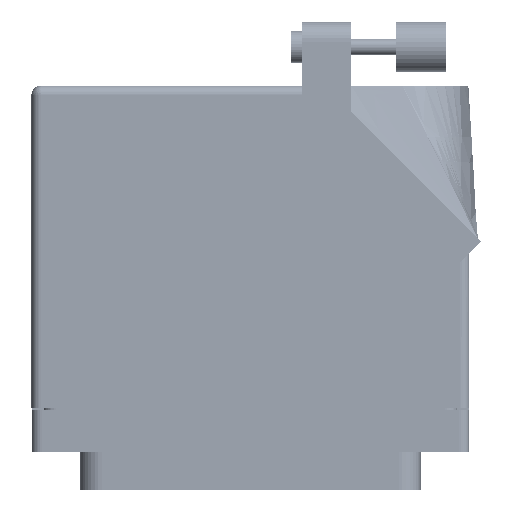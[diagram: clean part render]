
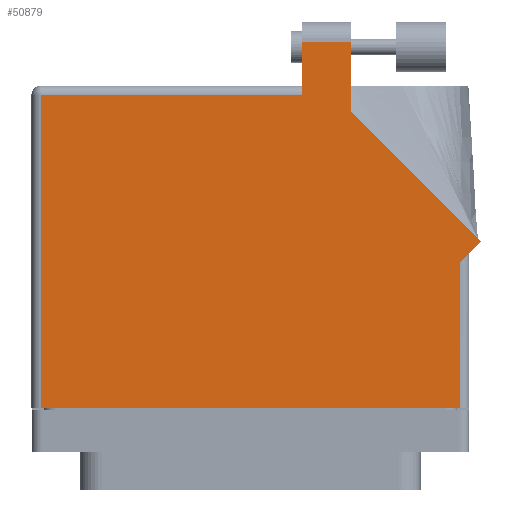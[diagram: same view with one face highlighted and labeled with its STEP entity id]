
A CAD part, front view. The second image highlights one B-rep face of the part: STEP entity #50879.
In plain terms, the highlighted face is planar.
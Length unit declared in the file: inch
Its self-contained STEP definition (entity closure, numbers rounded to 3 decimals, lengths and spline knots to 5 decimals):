
#1289 = VECTOR ( 'NONE', #21052, 39.37008 ) ;
#1736 = DIRECTION ( 'NONE',  ( 0., 1., 0. ) ) ;
#1799 = CARTESIAN_POINT ( 'NONE',  ( -1.3155, -0.1, 0.765 ) ) ;
#4821 = EDGE_CURVE ( 'NONE', #65087, #63755, #14002, .T. ) ;
#5730 = ORIENTED_EDGE ( 'NONE', *, *, #4821, .T. ) ;
#5805 = DIRECTION ( 'NONE',  ( -1., 0., 0. ) ) ;
#8644 = CARTESIAN_POINT ( 'NONE',  ( 0.6345, 1.76442, 0.765 ) ) ;
#9148 = VECTOR ( 'NONE', #45414, 39.37008 ) ;
#10805 = VERTEX_POINT ( 'NONE', #79497 ) ;
#12740 = LINE ( 'NONE', #88213, #39972 ) ;
#12773 = EDGE_CURVE ( 'NONE', #34754, #37723, #15149, .T. ) ;
#13889 = LINE ( 'NONE', #42337, #24087 ) ;
#14002 = LINE ( 'NONE', #1799, #28987 ) ;
#15149 = LINE ( 'NONE', #49030, #1289 ) ;
#16421 = EDGE_CURVE ( 'NONE', #44333, #29971, #66097, .T. ) ;
#19986 = CARTESIAN_POINT ( 'NONE',  ( -1.3155, -0.1, 0.765 ) ) ;
#21052 = DIRECTION ( 'NONE',  ( 0.707, 0.707, 0. ) ) ;
#21336 = CARTESIAN_POINT ( 'NONE',  ( -1.3155, 1.868, 0.765 ) ) ;
#22315 = ORIENTED_EDGE ( 'NONE', *, *, #12773, .T. ) ;
#22986 = LINE ( 'NONE', #49618, #57344 ) ;
#23316 = VECTOR ( 'NONE', #5805, 39.37008 ) ;
#23936 = CARTESIAN_POINT ( 'NONE',  ( 0.6345, 1.76442, 0.765 ) ) ;
#24087 = VECTOR ( 'NONE', #69951, 39.37008 ) ;
#27228 = DIRECTION ( 'NONE',  ( -1., 0., 0. ) ) ;
#28310 = VERTEX_POINT ( 'NONE', #46020 ) ;
#28943 = ORIENTED_EDGE ( 'NONE', *, *, #55375, .T. ) ;
#28987 = VECTOR ( 'NONE', #63258, 39.37008 ) ;
#29317 = LINE ( 'NONE', #36082, #59808 ) ;
#29971 = VERTEX_POINT ( 'NONE', #63590 ) ;
#33529 = CARTESIAN_POINT ( 'NONE',  ( -1.3775, 1.93, 0.765 ) ) ;
#34754 = VERTEX_POINT ( 'NONE', #73357 ) ;
#36082 = CARTESIAN_POINT ( 'NONE',  ( 1.3155, 0.88, 0.765 ) ) ;
#37723 = VERTEX_POINT ( 'NONE', #46540 ) ;
#39326 = VECTOR ( 'NONE', #43794, 39.37008 ) ;
#39972 = VECTOR ( 'NONE', #27228, 39.37008 ) ;
#42337 = CARTESIAN_POINT ( 'NONE',  ( 0.3275, 1.93, 0.765 ) ) ;
#42959 = EDGE_CURVE ( 'NONE', #29971, #10805, #13889, .T. ) ;
#43794 = DIRECTION ( 'NONE',  ( 0., 1., 0. ) ) ;
#44333 = VERTEX_POINT ( 'NONE', #65843 ) ;
#45414 = DIRECTION ( 'NONE',  ( -0.707, 0.707, 0. ) ) ;
#46020 = CARTESIAN_POINT ( 'NONE',  ( 1.3155, -0.1, 0.765 ) ) ;
#46540 = CARTESIAN_POINT ( 'NONE',  ( 1.44821, 0.95071, 0.765 ) ) ;
#48253 = ORIENTED_EDGE ( 'NONE', *, *, #80389, .T. ) ;
#49030 = CARTESIAN_POINT ( 'NONE',  ( 1.3775, 0.88, 0.765 ) ) ;
#49301 = ORIENTED_EDGE ( 'NONE', *, *, #16421, .T. ) ;
#49618 = CARTESIAN_POINT ( 'NONE',  ( -1.3775, -0.1, 0.765 ) ) ;
#50879 = ADVANCED_FACE ( 'NONE', ( #54762 ), #67886, .F. ) ;
#54762 = FACE_OUTER_BOUND ( 'NONE', #59839, .T. ) ;
#55375 = EDGE_CURVE ( 'NONE', #85901, #44333, #57366, .T. ) ;
#55625 = ORIENTED_EDGE ( 'NONE', *, *, #42959, .T. ) ;
#55938 = CARTESIAN_POINT ( 'NONE',  ( 0.3275, 2.205, 0.765 ) ) ;
#57344 = VECTOR ( 'NONE', #63188, 39.37008 ) ;
#57366 = LINE ( 'NONE', #23936, #39326 ) ;
#59808 = VECTOR ( 'NONE', #1736, 39.37008 ) ;
#59839 = EDGE_LOOP ( 'NONE', ( #28943, #49301, #55625, #69743, #5730, #48253, #79335, #22315, #82988 ) ) ;
#61105 = DIRECTION ( 'NONE',  ( 0., 0., -1. ) ) ;
#63188 = DIRECTION ( 'NONE',  ( 1., 0., 0. ) ) ;
#63258 = DIRECTION ( 'NONE',  ( 0., -1., 0. ) ) ;
#63590 = CARTESIAN_POINT ( 'NONE',  ( 0.3275, 2.205, 0.765 ) ) ;
#63755 = VERTEX_POINT ( 'NONE', #19986 ) ;
#65087 = VERTEX_POINT ( 'NONE', #21336 ) ;
#65326 = CARTESIAN_POINT ( 'NONE',  ( 1.44821, 0.95071, 0.765 ) ) ;
#65843 = CARTESIAN_POINT ( 'NONE',  ( 0.6345, 2.205, 0.765 ) ) ;
#66097 = LINE ( 'NONE', #55938, #23316 ) ;
#66651 = LINE ( 'NONE', #65326, #9148 ) ;
#67886 = PLANE ( 'NONE',  #77908 ) ;
#69743 = ORIENTED_EDGE ( 'NONE', *, *, #78409, .T. ) ;
#69951 = DIRECTION ( 'NONE',  ( 0., -1., 0. ) ) ;
#73357 = CARTESIAN_POINT ( 'NONE',  ( 1.3155, 0.818, 0.765 ) ) ;
#77908 = AXIS2_PLACEMENT_3D ( 'NONE', #33529, #61105, #82344 ) ;
#78409 = EDGE_CURVE ( 'NONE', #10805, #65087, #12740, .T. ) ;
#79335 = ORIENTED_EDGE ( 'NONE', *, *, #88287, .T. ) ;
#79497 = CARTESIAN_POINT ( 'NONE',  ( 0.3275, 1.868, 0.765 ) ) ;
#80389 = EDGE_CURVE ( 'NONE', #63755, #28310, #22986, .T. ) ;
#82344 = DIRECTION ( 'NONE',  ( -1., 0., 0. ) ) ;
#82988 = ORIENTED_EDGE ( 'NONE', *, *, #87577, .T. ) ;
#85901 = VERTEX_POINT ( 'NONE', #8644 ) ;
#87577 = EDGE_CURVE ( 'NONE', #37723, #85901, #66651, .T. ) ;
#88213 = CARTESIAN_POINT ( 'NONE',  ( -1.3775, 1.868, 0.765 ) ) ;
#88287 = EDGE_CURVE ( 'NONE', #28310, #34754, #29317, .T. ) ;
